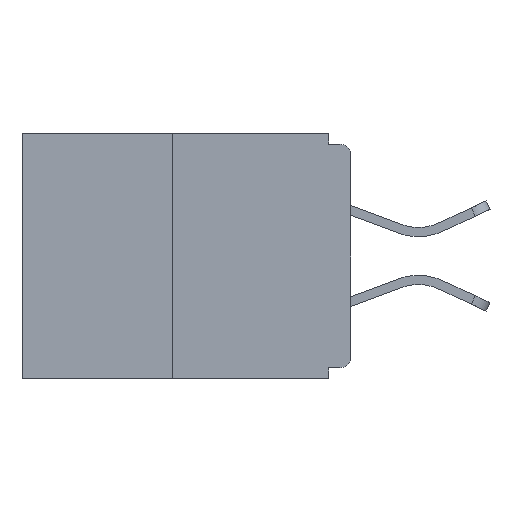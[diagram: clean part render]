
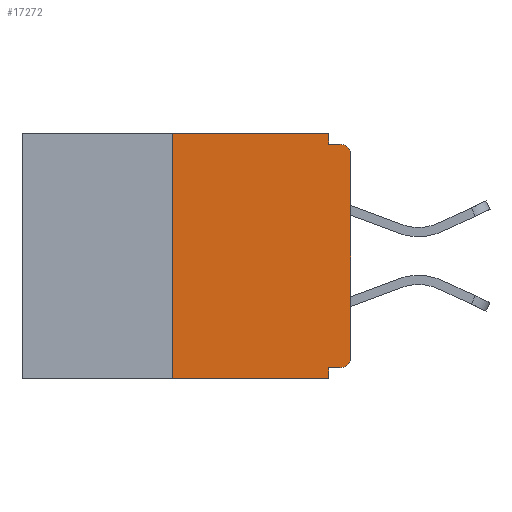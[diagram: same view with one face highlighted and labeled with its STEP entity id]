
A CAD part, left-side view. The second image highlights one B-rep face of the part: STEP entity #17272.
In plain terms, the highlighted planar face has unit normal (-1, 0, 0).
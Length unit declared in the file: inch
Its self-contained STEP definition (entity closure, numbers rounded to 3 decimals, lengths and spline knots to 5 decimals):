
#327 = DIRECTION ( 'NONE',  ( 0., 0., 1. ) ) ;
#810 = CARTESIAN_POINT ( 'NONE',  ( 0., 0.46, 0. ) ) ;
#1612 = ORIENTED_EDGE ( 'NONE', *, *, #10360, .F. ) ;
#1775 = LINE ( 'NONE', #19614, #17124 ) ;
#2051 = EDGE_CURVE ( 'NONE', #3730, #22978, #8796, .T. ) ;
#2100 = CARTESIAN_POINT ( 'NONE',  ( 0., 0.25, 0. ) ) ;
#2468 = VERTEX_POINT ( 'NONE', #14668 ) ;
#2489 = ORIENTED_EDGE ( 'NONE', *, *, #2051, .T. ) ;
#2551 = CARTESIAN_POINT ( 'NONE',  ( 0., 0., -0.03 ) ) ;
#2609 = ORIENTED_EDGE ( 'NONE', *, *, #14458, .F. ) ;
#2906 = VERTEX_POINT ( 'NONE', #4007 ) ;
#2960 = CARTESIAN_POINT ( 'NONE',  ( 0., 0.46, -0.343 ) ) ;
#3012 = VECTOR ( 'NONE', #327, 39.37008 ) ;
#3149 = CARTESIAN_POINT ( 'NONE',  ( 0., 0.031, 0. ) ) ;
#3489 = LINE ( 'NONE', #5344, #20689 ) ;
#3730 = VERTEX_POINT ( 'NONE', #8281 ) ;
#4007 = CARTESIAN_POINT ( 'NONE',  ( 0., 0.015, -0.328 ) ) ;
#4165 = ORIENTED_EDGE ( 'NONE', *, *, #13253, .F. ) ;
#4370 = LINE ( 'NONE', #19888, #6822 ) ;
#5344 = CARTESIAN_POINT ( 'NONE',  ( 0., 0., -0.015 ) ) ;
#5609 = ORIENTED_EDGE ( 'NONE', *, *, #12039, .T. ) ;
#5629 = DIRECTION ( 'NONE',  ( 0., 0., 1. ) ) ;
#6652 = EDGE_CURVE ( 'NONE', #22978, #11678, #15756, .T. ) ;
#6822 = VECTOR ( 'NONE', #16864, 39.37008 ) ;
#7036 = CARTESIAN_POINT ( 'NONE',  ( 0., 0., 0. ) ) ;
#7515 = EDGE_CURVE ( 'NONE', #2468, #12126, #4370, .T. ) ;
#7549 = EDGE_CURVE ( 'NONE', #16222, #12126, #15346, .T. ) ;
#7873 = EDGE_CURVE ( 'NONE', #2906, #2468, #16602, .T. ) ;
#7898 = DIRECTION ( 'NONE',  ( 0., 0., -1. ) ) ;
#8281 = CARTESIAN_POINT ( 'NONE',  ( 0., 0., -0.313 ) ) ;
#8366 = FACE_OUTER_BOUND ( 'NONE', #22818, .T. ) ;
#8796 = LINE ( 'NONE', #7036, #12541 ) ;
#8872 = DIRECTION ( 'NONE',  ( 0., -1., 0. ) ) ;
#9455 = ORIENTED_EDGE ( 'NONE', *, *, #7515, .F. ) ;
#10360 = EDGE_CURVE ( 'NONE', #12782, #16239, #1775, .T. ) ;
#10896 = AXIS2_PLACEMENT_3D ( 'NONE', #11178, #16575, #13045 ) ;
#11152 = CARTESIAN_POINT ( 'NONE',  ( 0., 0.25, 0. ) ) ;
#11178 = CARTESIAN_POINT ( 'NONE',  ( 0., 0.015, -0.03 ) ) ;
#11187 = AXIS2_PLACEMENT_3D ( 'NONE', #14653, #20371, #14882 ) ;
#11353 = ORIENTED_EDGE ( 'NONE', *, *, #6652, .T. ) ;
#11496 = CARTESIAN_POINT ( 'NONE',  ( 0., 0.031, -0.343 ) ) ;
#11678 = VERTEX_POINT ( 'NONE', #16234 ) ;
#11792 = ORIENTED_EDGE ( 'NONE', *, *, #7873, .F. ) ;
#12039 = EDGE_CURVE ( 'NONE', #2906, #3730, #18272, .T. ) ;
#12126 = VERTEX_POINT ( 'NONE', #11496 ) ;
#12541 = VECTOR ( 'NONE', #5629, 39.37008 ) ;
#12782 = VERTEX_POINT ( 'NONE', #2100 ) ;
#12908 = LINE ( 'NONE', #11152, #3012 ) ;
#13045 = DIRECTION ( 'NONE',  ( 0., 0., -1. ) ) ;
#13253 = EDGE_CURVE ( 'NONE', #16222, #12782, #12908, .T. ) ;
#13985 = DIRECTION ( 'NONE',  ( 0., 0., -1. ) ) ;
#14458 = EDGE_CURVE ( 'NONE', #16239, #20559, #15969, .T. ) ;
#14653 = CARTESIAN_POINT ( 'NONE',  ( 0., 0.015, -0.313 ) ) ;
#14660 = CARTESIAN_POINT ( 'NONE',  ( 0., 0.031, 0. ) ) ;
#14668 = CARTESIAN_POINT ( 'NONE',  ( 0., 0.031, -0.328 ) ) ;
#14882 = DIRECTION ( 'NONE',  ( 0., 0., -1. ) ) ;
#15346 = LINE ( 'NONE', #2960, #21756 ) ;
#15756 = CIRCLE ( 'NONE', #10896, 0.015 ) ;
#15969 = LINE ( 'NONE', #3149, #18328 ) ;
#16222 = VERTEX_POINT ( 'NONE', #21799 ) ;
#16234 = CARTESIAN_POINT ( 'NONE',  ( 0., 0.015, -0.015 ) ) ;
#16239 = VERTEX_POINT ( 'NONE', #14660 ) ;
#16479 = DIRECTION ( 'NONE',  ( 0., 1., 0. ) ) ;
#16575 = DIRECTION ( 'NONE',  ( -1., 0., 0. ) ) ;
#16602 = LINE ( 'NONE', #18572, #18392 ) ;
#16864 = DIRECTION ( 'NONE',  ( 0., 0., -1. ) ) ;
#16983 = DIRECTION ( 'NONE',  ( 0., -1., 0. ) ) ;
#17124 = VECTOR ( 'NONE', #8872, 39.37008 ) ;
#17254 = DIRECTION ( 'NONE',  ( 1., 0., 0. ) ) ;
#17272 = ADVANCED_FACE ( 'NONE', ( #8366 ), #22178, .F. ) ;
#17491 = DIRECTION ( 'NONE',  ( 0., -1., 0. ) ) ;
#18272 = CIRCLE ( 'NONE', #11187, 0.015 ) ;
#18328 = VECTOR ( 'NONE', #13985, 39.37008 ) ;
#18392 = VECTOR ( 'NONE', #16479, 39.37008 ) ;
#18456 = ORIENTED_EDGE ( 'NONE', *, *, #20935, .F. ) ;
#18572 = CARTESIAN_POINT ( 'NONE',  ( 0., 0., -0.328 ) ) ;
#19377 = CARTESIAN_POINT ( 'NONE',  ( 0., 0.031, -0.015 ) ) ;
#19614 = CARTESIAN_POINT ( 'NONE',  ( 0., 0.46, 0. ) ) ;
#19847 = ORIENTED_EDGE ( 'NONE', *, *, #7549, .T. ) ;
#19888 = CARTESIAN_POINT ( 'NONE',  ( 0., 0.031, -0.343 ) ) ;
#20178 = AXIS2_PLACEMENT_3D ( 'NONE', #810, #17254, #7898 ) ;
#20371 = DIRECTION ( 'NONE',  ( -1., 0., 0. ) ) ;
#20559 = VERTEX_POINT ( 'NONE', #19377 ) ;
#20689 = VECTOR ( 'NONE', #17491, 39.37008 ) ;
#20935 = EDGE_CURVE ( 'NONE', #20559, #11678, #3489, .T. ) ;
#21756 = VECTOR ( 'NONE', #16983, 39.37008 ) ;
#21799 = CARTESIAN_POINT ( 'NONE',  ( 0., 0.25, -0.343 ) ) ;
#22178 = PLANE ( 'NONE',  #20178 ) ;
#22818 = EDGE_LOOP ( 'NONE', ( #1612, #4165, #19847, #9455, #11792, #5609, #2489, #11353, #18456, #2609 ) ) ;
#22978 = VERTEX_POINT ( 'NONE', #2551 ) ;
